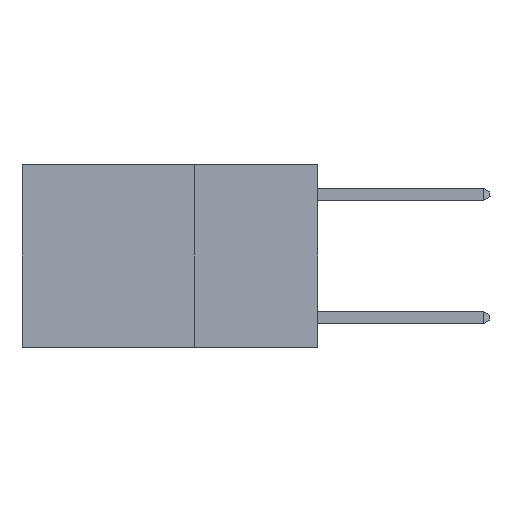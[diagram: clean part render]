
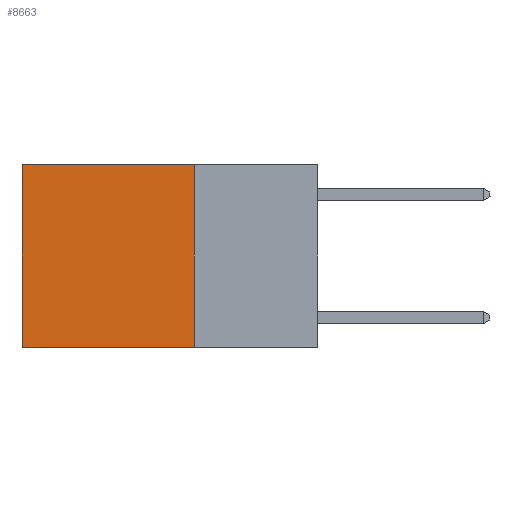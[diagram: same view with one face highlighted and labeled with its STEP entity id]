
A CAD part, left-side view. The second image highlights one B-rep face of the part: STEP entity #8663.
In plain terms, the highlighted planar face has unit normal (-1, 0, 0).
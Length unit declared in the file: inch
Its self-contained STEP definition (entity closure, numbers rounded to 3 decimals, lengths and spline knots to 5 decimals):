
#2052 = ORIENTED_EDGE ( 'NONE', *, *, #26334, .T. ) ;
#2107 = ORIENTED_EDGE ( 'NONE', *, *, #25771, .F. ) ;
#3253 = VERTEX_POINT ( 'NONE', #26688 ) ;
#4694 = VECTOR ( 'NONE', #8474, 39.37008 ) ;
#4798 = PLANE ( 'NONE',  #4937 ) ;
#4937 = AXIS2_PLACEMENT_3D ( 'NONE', #19296, #6949, #14228 ) ;
#5345 = EDGE_CURVE ( 'NONE', #3253, #17225, #7649, .T. ) ;
#6949 = DIRECTION ( 'NONE',  ( 1., 0., 0. ) ) ;
#7649 = LINE ( 'NONE', #14459, #21282 ) ;
#7999 = CARTESIAN_POINT ( 'NONE',  ( 0.2625, 0.6, -0.37 ) ) ;
#8368 = CARTESIAN_POINT ( 'NONE',  ( 0.2625, 0.25, 0. ) ) ;
#8474 = DIRECTION ( 'NONE',  ( 0., 1., 0. ) ) ;
#8554 = DIRECTION ( 'NONE',  ( 0., 0., -1. ) ) ;
#8663 = ADVANCED_FACE ( 'NONE', ( #19146 ), #4798, .F. ) ;
#9633 = DIRECTION ( 'NONE',  ( 0., 1., 0. ) ) ;
#13741 = CARTESIAN_POINT ( 'NONE',  ( 0.2625, 0.25, -0.37 ) ) ;
#14228 = DIRECTION ( 'NONE',  ( 0., 0., -1. ) ) ;
#14459 = CARTESIAN_POINT ( 'NONE',  ( 0.2625, 0.6, 0. ) ) ;
#14948 = VERTEX_POINT ( 'NONE', #30049 ) ;
#16450 = DIRECTION ( 'NONE',  ( 0., 0., -1. ) ) ;
#17225 = VERTEX_POINT ( 'NONE', #7999 ) ;
#18019 = VECTOR ( 'NONE', #8554, 39.37008 ) ;
#19146 = FACE_OUTER_BOUND ( 'NONE', #21585, .T. ) ;
#19296 = CARTESIAN_POINT ( 'NONE',  ( 0.2625, 0.25, 0. ) ) ;
#19619 = ORIENTED_EDGE ( 'NONE', *, *, #5345, .T. ) ;
#20845 = VERTEX_POINT ( 'NONE', #8368 ) ;
#21282 = VECTOR ( 'NONE', #16450, 39.37008 ) ;
#21517 = CARTESIAN_POINT ( 'NONE',  ( 0.2625, 0.25, 0. ) ) ;
#21585 = EDGE_LOOP ( 'NONE', ( #19619, #2107, #29223, #2052 ) ) ;
#21989 = VECTOR ( 'NONE', #9633, 39.37008 ) ;
#23527 = LINE ( 'NONE', #21517, #21989 ) ;
#25000 = LINE ( 'NONE', #13741, #4694 ) ;
#25771 = EDGE_CURVE ( 'NONE', #14948, #17225, #25000, .T. ) ;
#26018 = EDGE_CURVE ( 'NONE', #20845, #14948, #27080, .T. ) ;
#26334 = EDGE_CURVE ( 'NONE', #20845, #3253, #23527, .T. ) ;
#26688 = CARTESIAN_POINT ( 'NONE',  ( 0.2625, 0.6, 0. ) ) ;
#27080 = LINE ( 'NONE', #29251, #18019 ) ;
#29223 = ORIENTED_EDGE ( 'NONE', *, *, #26018, .F. ) ;
#29251 = CARTESIAN_POINT ( 'NONE',  ( 0.2625, 0.25, 0. ) ) ;
#30049 = CARTESIAN_POINT ( 'NONE',  ( 0.2625, 0.25, -0.37 ) ) ;
